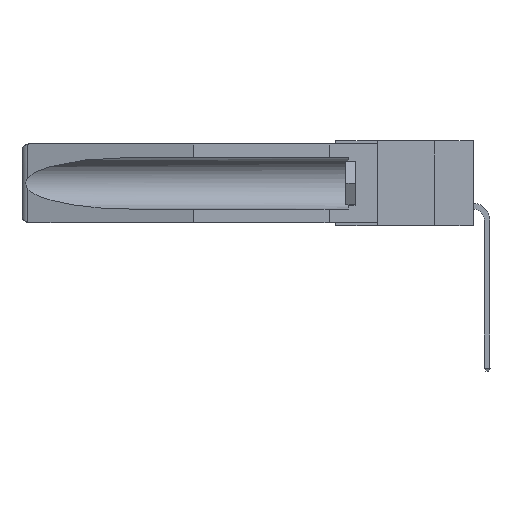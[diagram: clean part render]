
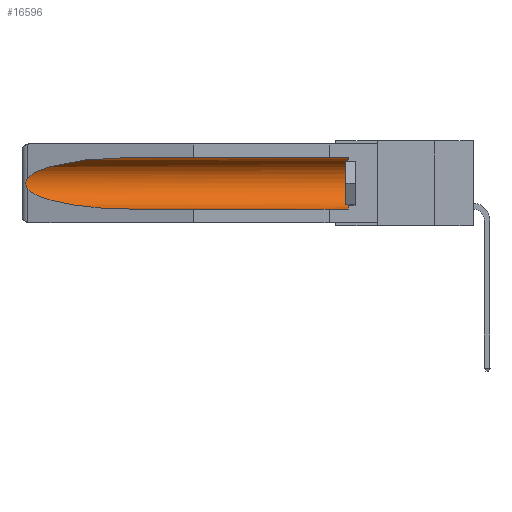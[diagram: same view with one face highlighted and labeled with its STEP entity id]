
A CAD part, left-side view. The second image highlights one B-rep face of the part: STEP entity #16596.
In plain terms, the highlighted cylindrical face has radius 2.857 mm (diameter 5.715 mm), a partial arc.
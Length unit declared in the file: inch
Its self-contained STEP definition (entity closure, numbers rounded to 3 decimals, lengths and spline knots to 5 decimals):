
#71 = EDGE_CURVE ( 'NONE', #14310, #9864, #29803, .T. ) ;
#88 = DIRECTION ( 'NONE',  ( 0., 1., 0. ) ) ;
#273 = EDGE_CURVE ( 'NONE', #9864, #25842, #6668, .T. ) ;
#1479 = CARTESIAN_POINT ( 'NONE',  ( 0.26537, 1.52718, -0.19328 ) ) ;
#1591 = CARTESIAN_POINT ( 'NONE',  ( 0.155, 1.07973, -0.284 ) ) ;
#1797 = CARTESIAN_POINT ( 'NONE',  ( 0.155, -0.30754, -0.1715 ) ) ;
#2281 = CARTESIAN_POINT ( 'NONE',  ( 0.155, 0.126, -0.059 ) ) ;
#2775 = CARTESIAN_POINT ( 'NONE',  ( 0.2673, 1.5327, -0.16383 ) ) ;
#3065 = AXIS2_PLACEMENT_3D ( 'NONE', #14006, #12106, #30075 ) ;
#3328 = CARTESIAN_POINT ( 'NONE',  ( 0.155, 1.07973, -0.059 ) ) ;
#3469 = VERTEX_POINT ( 'NONE', #2281 ) ;
#3706 = EDGE_CURVE ( 'NONE', #27926, #14310, #14269, .T. ) ;
#3840 = CARTESIAN_POINT ( 'NONE',  ( 0.25451, 1.48313, -0.24835 ) ) ;
#5033 = CARTESIAN_POINT ( 'NONE',  ( 0.26537, 1.52718, -0.19328 ) ) ;
#5763 = DIRECTION ( 'NONE',  ( 0., 1., 0. ) ) ;
#5793 = CARTESIAN_POINT ( 'NONE',  ( 0.26654, 1.53092, -0.15636 ) ) ;
#5984 = VERTEX_POINT ( 'NONE', #29514 ) ;
#6668 =( BOUNDED_CURVE ( )  B_SPLINE_CURVE ( 3, ( #1479, #3840, #10607, #1591 ),
 .UNSPECIFIED., .F., .F. ) 
 B_SPLINE_CURVE_WITH_KNOTS ( ( 4, 4 ),
 ( 0.1948, 1.5708 ),
 .UNSPECIFIED. ) 
 CURVE ( )  GEOMETRIC_REPRESENTATION_ITEM ( )  RATIONAL_B_SPLINE_CURVE ( ( 1., 0.848, 0.848, 1. ) ) 
 REPRESENTATION_ITEM ( '' )  );
#7872 = ORIENTED_EDGE ( 'NONE', *, *, #273, .T. ) ;
#7957 = CARTESIAN_POINT ( 'NONE',  ( 0.2673, 1.53269, -0.17917 ) ) ;
#8001 = ORIENTED_EDGE ( 'NONE', *, *, #16778, .T. ) ;
#8659 = CARTESIAN_POINT ( 'NONE',  ( 0.26537, 1.52718, -0.14972 ) ) ;
#9346 = CARTESIAN_POINT ( 'NONE',  ( 0.155, 1.07973, -0.059 ) ) ;
#9864 = VERTEX_POINT ( 'NONE', #5033 ) ;
#9953 = VECTOR ( 'NONE', #88, 39.37008 ) ;
#10153 = CARTESIAN_POINT ( 'NONE',  ( 0.2675, 1.53308, -0.16763 ) ) ;
#10375 = ORIENTED_EDGE ( 'NONE', *, *, #26735, .F. ) ;
#10607 = CARTESIAN_POINT ( 'NONE',  ( 0.21114, 1.30732, -0.284 ) ) ;
#10683 = CARTESIAN_POINT ( 'NONE',  ( 0.2675, 1.53308, -0.17534 ) ) ;
#11482 = CYLINDRICAL_SURFACE ( 'NONE', #30855, 0.1125 ) ;
#12106 = DIRECTION ( 'NONE',  ( 0., -1., 0. ) ) ;
#14006 = CARTESIAN_POINT ( 'NONE',  ( 0.155, 0.126, -0.1715 ) ) ;
#14269 =( BOUNDED_CURVE ( )  B_SPLINE_CURVE ( 3, ( #3328, #27669, #25184, #24969 ),
 .UNSPECIFIED., .F., .F. ) 
 B_SPLINE_CURVE_WITH_KNOTS ( ( 4, 4 ),
 ( 4.71239, 6.08839 ),
 .UNSPECIFIED. ) 
 CURVE ( )  GEOMETRIC_REPRESENTATION_ITEM ( )  RATIONAL_B_SPLINE_CURVE ( ( 1., 0.848, 0.848, 1. ) ) 
 REPRESENTATION_ITEM ( '' )  );
#14310 = VERTEX_POINT ( 'NONE', #15851 ) ;
#15020 = LINE ( 'NONE', #30144, #24035 ) ;
#15291 = ORIENTED_EDGE ( 'NONE', *, *, #31069, .T. ) ;
#15567 = ORIENTED_EDGE ( 'NONE', *, *, #3706, .T. ) ;
#15851 = CARTESIAN_POINT ( 'NONE',  ( 0.26537, 1.52718, -0.14972 ) ) ;
#16596 = ADVANCED_FACE ( 'NONE', ( #30823 ), #11482, .F. ) ;
#16778 = EDGE_CURVE ( 'NONE', #3469, #27926, #17530, .T. ) ;
#16908 = CARTESIAN_POINT ( 'NONE',  ( 0.26597, 1.52961, -0.15275 ) ) ;
#17494 = CARTESIAN_POINT ( 'NONE',  ( 0.26655, 1.53094, -0.18657 ) ) ;
#17530 = LINE ( 'NONE', #21878, #9953 ) ;
#18941 = DIRECTION ( 'NONE',  ( 0., 1., 0. ) ) ;
#19853 = EDGE_LOOP ( 'NONE', ( #15567, #22687, #7872, #10375, #15291, #8001 ) ) ;
#20033 = CARTESIAN_POINT ( 'NONE',  ( 0.26537, 1.52718, -0.19328 ) ) ;
#21878 = CARTESIAN_POINT ( 'NONE',  ( 0.155, -0.30754, -0.059 ) ) ;
#22263 = CIRCLE ( 'NONE', #3065, 0.1125 ) ;
#22687 = ORIENTED_EDGE ( 'NONE', *, *, #71, .T. ) ;
#24035 = VECTOR ( 'NONE', #5763, 39.37008 ) ;
#24969 = CARTESIAN_POINT ( 'NONE',  ( 0.26537, 1.52718, -0.14972 ) ) ;
#25184 = CARTESIAN_POINT ( 'NONE',  ( 0.25451, 1.48313, -0.09465 ) ) ;
#25842 = VERTEX_POINT ( 'NONE', #30178 ) ;
#26735 = EDGE_CURVE ( 'NONE', #5984, #25842, #15020, .T. ) ;
#27334 = CARTESIAN_POINT ( 'NONE',  ( 0.26597, 1.5296, -0.19026 ) ) ;
#27669 = CARTESIAN_POINT ( 'NONE',  ( 0.21114, 1.30732, -0.059 ) ) ;
#27926 = VERTEX_POINT ( 'NONE', #9346 ) ;
#28590 = DIRECTION ( 'NONE',  ( 0., 0., 1. ) ) ;
#29514 = CARTESIAN_POINT ( 'NONE',  ( 0.155, 0.126, -0.284 ) ) ;
#29803 = B_SPLINE_CURVE_WITH_KNOTS ( 'NONE', 3,
 ( #8659, #16908, #5793, #2775, #10153, #10683, #7957, #17494, #27334, #20033 ),
 .UNSPECIFIED., .F., .F.,
 ( 4, 2, 2, 2, 4 ),
 ( 0., 0.00029, 0.00058, 0.00087, 0.00117 ),
 .UNSPECIFIED. ) ;
#30075 = DIRECTION ( 'NONE',  ( 0., 0., 1. ) ) ;
#30144 = CARTESIAN_POINT ( 'NONE',  ( 0.155, -0.30754, -0.284 ) ) ;
#30178 = CARTESIAN_POINT ( 'NONE',  ( 0.155, 1.07973, -0.284 ) ) ;
#30823 = FACE_OUTER_BOUND ( 'NONE', #19853, .T. ) ;
#30855 = AXIS2_PLACEMENT_3D ( 'NONE', #1797, #18941, #28590 ) ;
#31069 = EDGE_CURVE ( 'NONE', #5984, #3469, #22263, .T. ) ;
